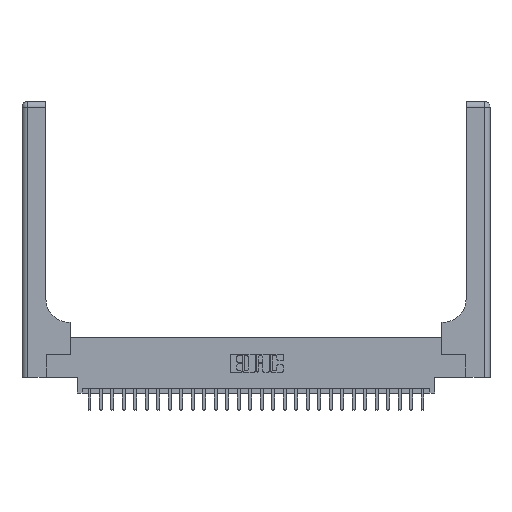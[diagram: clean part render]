
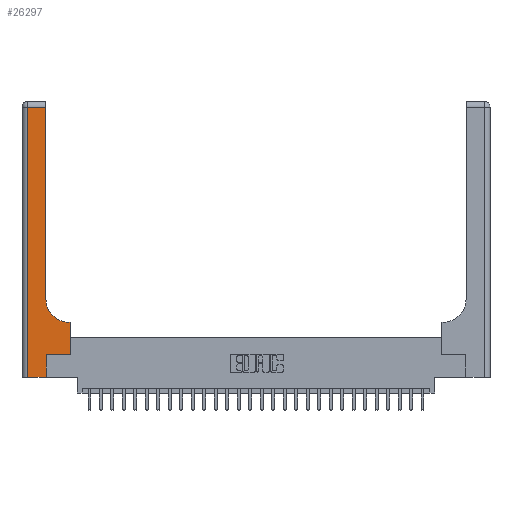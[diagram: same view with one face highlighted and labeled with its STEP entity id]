
A CAD part, top view. The second image highlights one B-rep face of the part: STEP entity #26297.
In plain terms, the highlighted planar face has unit normal (0, 0, 1).
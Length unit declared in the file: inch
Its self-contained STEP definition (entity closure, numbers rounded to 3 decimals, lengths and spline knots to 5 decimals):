
#451 = ORIENTED_EDGE ( 'NONE', *, *, #19786, .T. ) ;
#625 = ORIENTED_EDGE ( 'NONE', *, *, #26260, .T. ) ;
#675 = ORIENTED_EDGE ( 'NONE', *, *, #24906, .T. ) ;
#879 = ORIENTED_EDGE ( 'NONE', *, *, #13634, .T. ) ;
#931 = ORIENTED_EDGE ( 'NONE', *, *, #25056, .T. ) ;
#1068 = EDGE_CURVE ( 'NONE', #12418, #19282, #4506, .T. ) ;
#1856 = VERTEX_POINT ( 'NONE', #10096 ) ;
#2527 = VERTEX_POINT ( 'NONE', #6001 ) ;
#3309 = VERTEX_POINT ( 'NONE', #16282 ) ;
#3851 = CARTESIAN_POINT ( 'NONE',  ( 0.265, 0.25, 0.37 ) ) ;
#4440 = CIRCLE ( 'NONE', #23634, 0.25 ) ;
#4506 = LINE ( 'NONE', #21366, #5139 ) ;
#4630 = EDGE_LOOP ( 'NONE', ( #21277, #21477, #12707, #25513, #451, #625, #675, #879, #931 ) ) ;
#5139 = VECTOR ( 'NONE', #26343, 39.37008 ) ;
#5253 = EDGE_CURVE ( 'NONE', #22317, #12418, #20837, .T. ) ;
#5338 = CARTESIAN_POINT ( 'NONE',  ( 0.26, 3., 0.37 ) ) ;
#6001 = CARTESIAN_POINT ( 'NONE',  ( 0.26, 0.85, 0.37 ) ) ;
#6019 = CARTESIAN_POINT ( 'NONE',  ( 0.528, 0.25, 0.37 ) ) ;
#6330 = FACE_OUTER_BOUND ( 'NONE', #4630, .T. ) ;
#7319 = LINE ( 'NONE', #6019, #13468 ) ;
#7439 = DIRECTION ( 'NONE',  ( 0., 1., 0. ) ) ;
#8053 = CARTESIAN_POINT ( 'NONE',  ( 0., 0., 0.37 ) ) ;
#8100 = DIRECTION ( 'NONE',  ( 0., 1., 0. ) ) ;
#8219 = PLANE ( 'NONE',  #12891 ) ;
#8272 = VECTOR ( 'NONE', #10126, 39.37008 ) ;
#8469 = DIRECTION ( 'NONE',  ( 0., 0., -1. ) ) ;
#8650 = CARTESIAN_POINT ( 'NONE',  ( 0.528, 0.6, 0.37 ) ) ;
#9950 = CARTESIAN_POINT ( 'NONE',  ( 0.265, 0., 0.37 ) ) ;
#10045 = CARTESIAN_POINT ( 'NONE',  ( 0.06, 2.94, 0.37 ) ) ;
#10096 = CARTESIAN_POINT ( 'NONE',  ( 0.265, 0.25, 0.37 ) ) ;
#10126 = DIRECTION ( 'NONE',  ( 1., 0., 0. ) ) ;
#10528 = DIRECTION ( 'NONE',  ( -1., 0., 0. ) ) ;
#10541 = CARTESIAN_POINT ( 'NONE',  ( 0.06, 0., 0.37 ) ) ;
#11868 = VECTOR ( 'NONE', #7439, 39.37008 ) ;
#12022 = DIRECTION ( 'NONE',  ( 0., 1., 0. ) ) ;
#12380 = CARTESIAN_POINT ( 'NONE',  ( 0., 3., 0.37 ) ) ;
#12418 = VERTEX_POINT ( 'NONE', #10045 ) ;
#12422 = EDGE_CURVE ( 'NONE', #19282, #3309, #15778, .T. ) ;
#12539 = LINE ( 'NONE', #5338, #11868 ) ;
#12707 = ORIENTED_EDGE ( 'NONE', *, *, #1068, .T. ) ;
#12891 = AXIS2_PLACEMENT_3D ( 'NONE', #12380, #26621, #14453 ) ;
#13468 = VECTOR ( 'NONE', #8100, 39.37008 ) ;
#13634 = EDGE_CURVE ( 'NONE', #18756, #21870, #20206, .T. ) ;
#14274 = DIRECTION ( 'NONE',  ( 1., 0., 0. ) ) ;
#14453 = DIRECTION ( 'NONE',  ( -1., 0., 0. ) ) ;
#15778 = LINE ( 'NONE', #8053, #16451 ) ;
#16282 = CARTESIAN_POINT ( 'NONE',  ( 0.265, 0., 0.37 ) ) ;
#16451 = VECTOR ( 'NONE', #14274, 39.37008 ) ;
#17320 = CARTESIAN_POINT ( 'NONE',  ( 0.528, 0.25, 0.37 ) ) ;
#18580 = LINE ( 'NONE', #3851, #8272 ) ;
#18692 = VECTOR ( 'NONE', #12022, 39.37008 ) ;
#18756 = VERTEX_POINT ( 'NONE', #8650 ) ;
#18952 = CARTESIAN_POINT ( 'NONE',  ( 0.51, 0.6, 0.37 ) ) ;
#19282 = VERTEX_POINT ( 'NONE', #10541 ) ;
#19338 = LINE ( 'NONE', #9950, #18692 ) ;
#19564 = VECTOR ( 'NONE', #24598, 39.37008 ) ;
#19786 = EDGE_CURVE ( 'NONE', #3309, #1856, #19338, .T. ) ;
#20072 = VERTEX_POINT ( 'NONE', #17320 ) ;
#20206 = LINE ( 'NONE', #22792, #25609 ) ;
#20770 = CARTESIAN_POINT ( 'NONE',  ( 0.51, 0.85, 0.37 ) ) ;
#20837 = LINE ( 'NONE', #24444, #19564 ) ;
#21277 = ORIENTED_EDGE ( 'NONE', *, *, #25396, .T. ) ;
#21366 = CARTESIAN_POINT ( 'NONE',  ( 0.06, 3., 0.37 ) ) ;
#21477 = ORIENTED_EDGE ( 'NONE', *, *, #5253, .T. ) ;
#21870 = VERTEX_POINT ( 'NONE', #18952 ) ;
#22287 = CARTESIAN_POINT ( 'NONE',  ( 0.26, 2.94, 0.37 ) ) ;
#22317 = VERTEX_POINT ( 'NONE', #22287 ) ;
#22792 = CARTESIAN_POINT ( 'NONE',  ( 0.26, 0.6, 0.37 ) ) ;
#22827 = DIRECTION ( 'NONE',  ( 1., 0., 0. ) ) ;
#23634 = AXIS2_PLACEMENT_3D ( 'NONE', #20770, #8469, #22827 ) ;
#24444 = CARTESIAN_POINT ( 'NONE',  ( 0., 2.94, 0.37 ) ) ;
#24598 = DIRECTION ( 'NONE',  ( -1., 0., 0. ) ) ;
#24906 = EDGE_CURVE ( 'NONE', #20072, #18756, #7319, .T. ) ;
#25056 = EDGE_CURVE ( 'NONE', #21870, #2527, #4440, .T. ) ;
#25396 = EDGE_CURVE ( 'NONE', #2527, #22317, #12539, .T. ) ;
#25513 = ORIENTED_EDGE ( 'NONE', *, *, #12422, .T. ) ;
#25609 = VECTOR ( 'NONE', #10528, 39.37008 ) ;
#26260 = EDGE_CURVE ( 'NONE', #1856, #20072, #18580, .T. ) ;
#26297 = ADVANCED_FACE ( 'NONE', ( #6330 ), #8219, .F. ) ;
#26343 = DIRECTION ( 'NONE',  ( 0., -1., 0. ) ) ;
#26621 = DIRECTION ( 'NONE',  ( 0., 0., -1. ) ) ;
